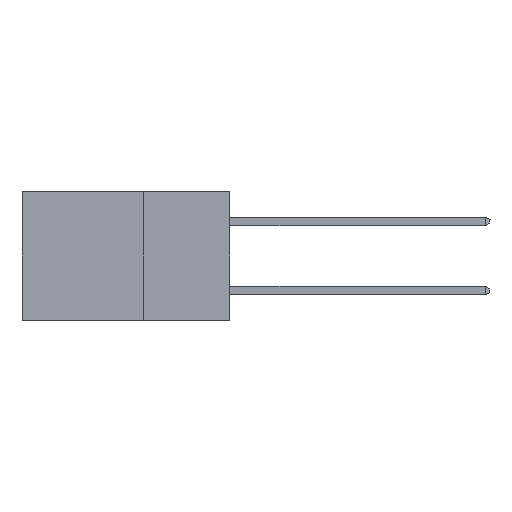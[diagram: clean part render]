
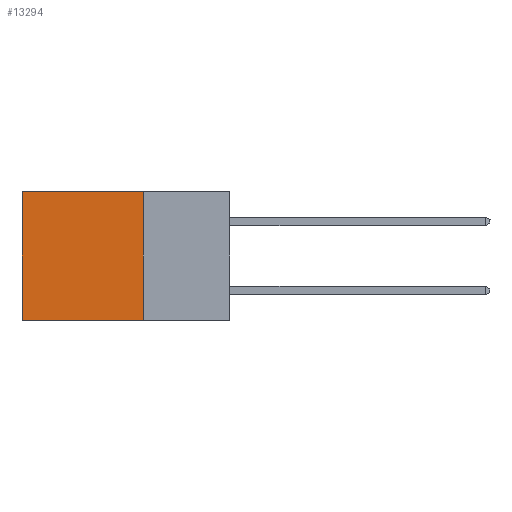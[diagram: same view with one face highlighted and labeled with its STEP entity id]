
A CAD part, left-side view. The second image highlights one B-rep face of the part: STEP entity #13294.
In plain terms, the highlighted planar face has unit normal (-1, 0, 0).
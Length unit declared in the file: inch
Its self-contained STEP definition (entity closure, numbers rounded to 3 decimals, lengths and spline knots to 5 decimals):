
#350 = AXIS2_PLACEMENT_3D ( 'NONE', #30051, #25103, #9556 ) ;
#1001 = VERTEX_POINT ( 'NONE', #18278 ) ;
#2069 = ORIENTED_EDGE ( 'NONE', *, *, #5218, .T. ) ;
#3021 = EDGE_CURVE ( 'NONE', #1001, #21408, #33565, .T. ) ;
#5018 = DIRECTION ( 'NONE',  ( 0., 1., 0. ) ) ;
#5218 = EDGE_CURVE ( 'NONE', #22107, #21408, #6072, .T. ) ;
#5817 = ORIENTED_EDGE ( 'NONE', *, *, #10538, .F. ) ;
#6072 = LINE ( 'NONE', #17555, #32085 ) ;
#6974 = CARTESIAN_POINT ( 'NONE',  ( 0.298, 0.25, 0. ) ) ;
#8750 = DIRECTION ( 'NONE',  ( 0., 0., -1. ) ) ;
#8769 = EDGE_CURVE ( 'NONE', #15601, #22107, #12907, .T. ) ;
#9556 = DIRECTION ( 'NONE',  ( 0., 0., -1. ) ) ;
#10304 = CARTESIAN_POINT ( 'NONE',  ( 0.298, 0.25, 0. ) ) ;
#10538 = EDGE_CURVE ( 'NONE', #15601, #1001, #11984, .T. ) ;
#11984 = LINE ( 'NONE', #6974, #25795 ) ;
#12811 = CARTESIAN_POINT ( 'NONE',  ( 0.298, 0.6, -0.37 ) ) ;
#12907 = LINE ( 'NONE', #18025, #19918 ) ;
#13294 = ADVANCED_FACE ( 'NONE', ( #19345 ), #19941, .F. ) ;
#13456 = CARTESIAN_POINT ( 'NONE',  ( 0.298, 0.6, 0. ) ) ;
#15601 = VERTEX_POINT ( 'NONE', #10304 ) ;
#17555 = CARTESIAN_POINT ( 'NONE',  ( 0.298, 0.6, 0. ) ) ;
#18025 = CARTESIAN_POINT ( 'NONE',  ( 0.298, 0.25, 0. ) ) ;
#18278 = CARTESIAN_POINT ( 'NONE',  ( 0.298, 0.25, -0.37 ) ) ;
#19345 = FACE_OUTER_BOUND ( 'NONE', #27817, .T. ) ;
#19918 = VECTOR ( 'NONE', #5018, 39.37008 ) ;
#19941 = PLANE ( 'NONE',  #350 ) ;
#20025 = VECTOR ( 'NONE', #27295, 39.37008 ) ;
#21408 = VERTEX_POINT ( 'NONE', #12811 ) ;
#22107 = VERTEX_POINT ( 'NONE', #13456 ) ;
#24259 = CARTESIAN_POINT ( 'NONE',  ( 0.298, 0.25, -0.37 ) ) ;
#25103 = DIRECTION ( 'NONE',  ( 1., 0., 0. ) ) ;
#25134 = DIRECTION ( 'NONE',  ( 0., 0., -1. ) ) ;
#25795 = VECTOR ( 'NONE', #25134, 39.37008 ) ;
#27295 = DIRECTION ( 'NONE',  ( 0., 1., 0. ) ) ;
#27817 = EDGE_LOOP ( 'NONE', ( #2069, #32312, #5817, #30828 ) ) ;
#30051 = CARTESIAN_POINT ( 'NONE',  ( 0.298, 0.25, 0. ) ) ;
#30828 = ORIENTED_EDGE ( 'NONE', *, *, #8769, .T. ) ;
#32085 = VECTOR ( 'NONE', #8750, 39.37008 ) ;
#32312 = ORIENTED_EDGE ( 'NONE', *, *, #3021, .F. ) ;
#33565 = LINE ( 'NONE', #24259, #20025 ) ;
